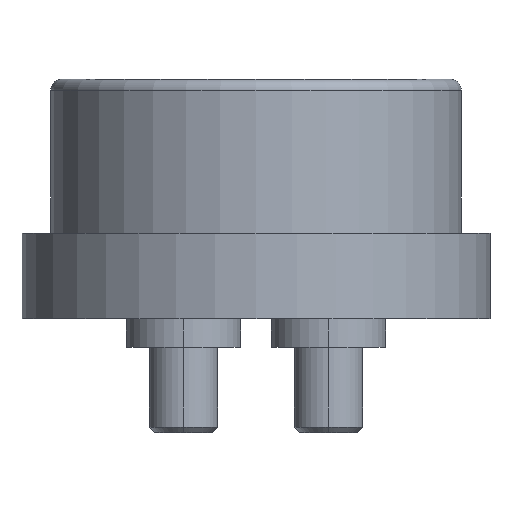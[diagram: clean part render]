
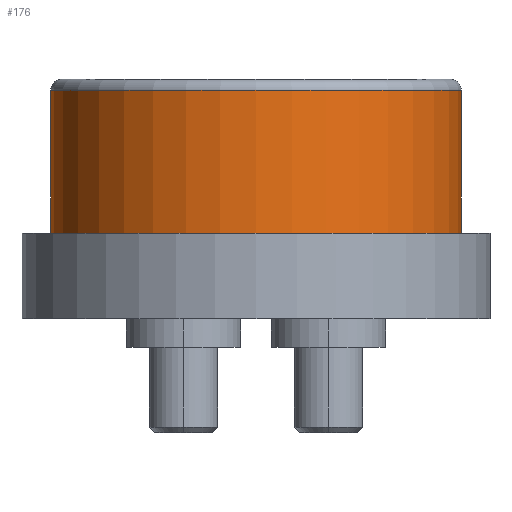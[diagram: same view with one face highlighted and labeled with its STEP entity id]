
A CAD part, left-side view. The second image highlights one B-rep face of the part: STEP entity #176.
In plain terms, the highlighted cylindrical face has radius 3.6 mm (diameter 7.2 mm), a partial arc.
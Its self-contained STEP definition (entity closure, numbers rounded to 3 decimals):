
#176 = ADVANCED_FACE ( 'NONE', ( #900 ), #1641, .T. ) ;
#377 = EDGE_CURVE ( 'NONE', #2059, #2649, #3969, .T. ) ;
#539 = DIRECTION ( 'NONE',  ( 0., 0., 1. ) ) ;
#713 = LINE ( 'NONE', #4602, #6994 ) ;
#900 = FACE_OUTER_BOUND ( 'NONE', #1976, .T. ) ;
#950 = DIRECTION ( 'NONE',  ( 0., 0., -1. ) ) ;
#1641 = CYLINDRICAL_SURFACE ( 'NONE', #4267, 3.6 ) ;
#1825 = DIRECTION ( 'NONE',  ( -1., 0., 0. ) ) ;
#1840 = EDGE_CURVE ( 'NONE', #2059, #8260, #2060, .T. ) ;
#1976 = EDGE_LOOP ( 'NONE', ( #3207, #8811, #4479, #2040 ) ) ;
#2040 = ORIENTED_EDGE ( 'NONE', *, *, #7313, .T. ) ;
#2059 = VERTEX_POINT ( 'NONE', #7323 ) ;
#2060 = LINE ( 'NONE', #4239, #3020 ) ;
#2168 = CARTESIAN_POINT ( 'NONE',  ( -8.35, -3.6, -12.7 ) ) ;
#2400 = AXIS2_PLACEMENT_3D ( 'NONE', #6912, #3986, #3838 ) ;
#2649 = VERTEX_POINT ( 'NONE', #2168 ) ;
#2714 = CARTESIAN_POINT ( 'NONE',  ( -8.35, 0., -10.2 ) ) ;
#3020 = VECTOR ( 'NONE', #539, 1000. ) ;
#3207 = ORIENTED_EDGE ( 'NONE', *, *, #1840, .F. ) ;
#3676 = EDGE_CURVE ( 'NONE', #7290, #2649, #713, .T. ) ;
#3838 = DIRECTION ( 'NONE',  ( -1., 0., 0. ) ) ;
#3905 = CARTESIAN_POINT ( 'NONE',  ( -8.35, 0., -10.15 ) ) ;
#3969 = CIRCLE ( 'NONE', #2400, 3.6 ) ;
#3986 = DIRECTION ( 'NONE',  ( 0., 0., 1. ) ) ;
#4239 = CARTESIAN_POINT ( 'NONE',  ( -8.35, 3.6, -12.7 ) ) ;
#4249 = CARTESIAN_POINT ( 'NONE',  ( -8.35, -3.6, -10.2 ) ) ;
#4267 = AXIS2_PLACEMENT_3D ( 'NONE', #3905, #950, #9153 ) ;
#4479 = ORIENTED_EDGE ( 'NONE', *, *, #3676, .F. ) ;
#4602 = CARTESIAN_POINT ( 'NONE',  ( -8.35, -3.6, -10.2 ) ) ;
#4694 = CIRCLE ( 'NONE', #8742, 3.6 ) ;
#5024 = CARTESIAN_POINT ( 'NONE',  ( -8.35, 3.6, -10.2 ) ) ;
#5695 = DIRECTION ( 'NONE',  ( 0., 0., -1. ) ) ;
#6912 = CARTESIAN_POINT ( 'NONE',  ( -8.35, 0., -12.7 ) ) ;
#6994 = VECTOR ( 'NONE', #9649, 1000. ) ;
#7290 = VERTEX_POINT ( 'NONE', #4249 ) ;
#7313 = EDGE_CURVE ( 'NONE', #7290, #8260, #4694, .T. ) ;
#7323 = CARTESIAN_POINT ( 'NONE',  ( -8.35, 3.6, -12.7 ) ) ;
#8260 = VERTEX_POINT ( 'NONE', #5024 ) ;
#8742 = AXIS2_PLACEMENT_3D ( 'NONE', #2714, #5695, #1825 ) ;
#8811 = ORIENTED_EDGE ( 'NONE', *, *, #377, .T. ) ;
#9153 = DIRECTION ( 'NONE',  ( 1., 0., 0. ) ) ;
#9649 = DIRECTION ( 'NONE',  ( 0., 0., -1. ) ) ;
